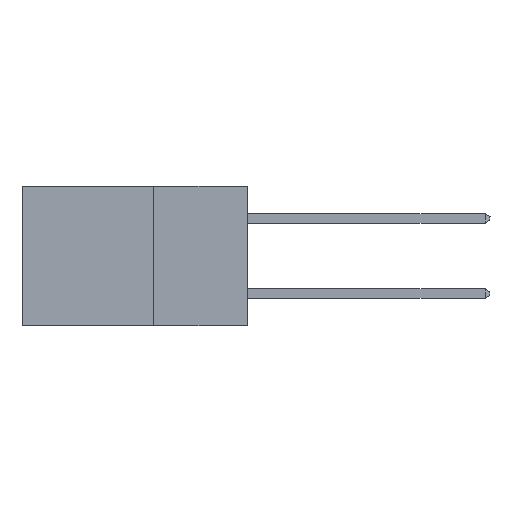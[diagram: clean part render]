
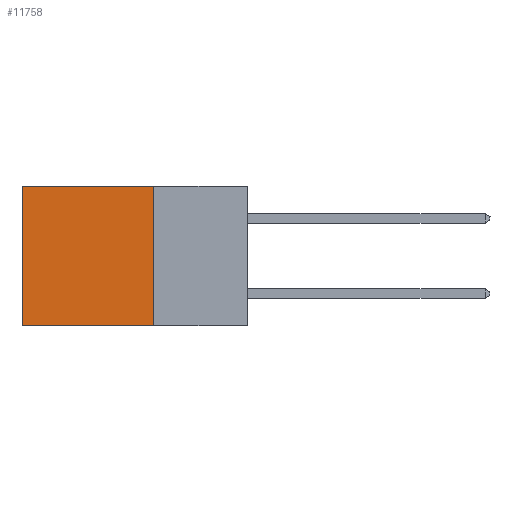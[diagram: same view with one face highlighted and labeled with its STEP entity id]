
A CAD part, left-side view. The second image highlights one B-rep face of the part: STEP entity #11758.
In plain terms, the highlighted planar face has unit normal (-1, 0, 0).
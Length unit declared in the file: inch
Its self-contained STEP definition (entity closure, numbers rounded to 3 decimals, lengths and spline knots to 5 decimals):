
#972 = DIRECTION ( 'NONE',  ( 0., 0., -1. ) ) ;
#1285 = EDGE_CURVE ( 'NONE', #8118, #17731, #5381, .T. ) ;
#1429 = LINE ( 'NONE', #10529, #5574 ) ;
#1528 = CARTESIAN_POINT ( 'NONE',  ( 0.2615, 0.25, 0. ) ) ;
#1572 = DIRECTION ( 'NONE',  ( 0., 0., -1. ) ) ;
#1685 = ORIENTED_EDGE ( 'NONE', *, *, #16047, .F. ) ;
#2729 = DIRECTION ( 'NONE',  ( 0., 1., 0. ) ) ;
#2750 = VECTOR ( 'NONE', #16886, 39.37008 ) ;
#2958 = PLANE ( 'NONE',  #10646 ) ;
#3011 = DIRECTION ( 'NONE',  ( 0., 1., 0. ) ) ;
#3368 = VERTEX_POINT ( 'NONE', #1528 ) ;
#3438 = EDGE_CURVE ( 'NONE', #3368, #5567, #10914, .T. ) ;
#4516 = CARTESIAN_POINT ( 'NONE',  ( 0.2615, 0.25, -0.37 ) ) ;
#5381 = LINE ( 'NONE', #16934, #14533 ) ;
#5567 = VERTEX_POINT ( 'NONE', #5978 ) ;
#5574 = VECTOR ( 'NONE', #3011, 39.37008 ) ;
#5978 = CARTESIAN_POINT ( 'NONE',  ( 0.2615, 0.25, -0.37 ) ) ;
#7473 = CARTESIAN_POINT ( 'NONE',  ( 0.2615, 0.6, -0.37 ) ) ;
#8118 = VERTEX_POINT ( 'NONE', #16156 ) ;
#8455 = ORIENTED_EDGE ( 'NONE', *, *, #3438, .F. ) ;
#8831 = FACE_OUTER_BOUND ( 'NONE', #18727, .T. ) ;
#10159 = CARTESIAN_POINT ( 'NONE',  ( 0.2615, 0.25, 0. ) ) ;
#10181 = DIRECTION ( 'NONE',  ( 1., 0., 0. ) ) ;
#10529 = CARTESIAN_POINT ( 'NONE',  ( 0.2615, 0.25, -0.37 ) ) ;
#10646 = AXIS2_PLACEMENT_3D ( 'NONE', #4516, #10181, #1572 ) ;
#10914 = LINE ( 'NONE', #18470, #2750 ) ;
#11339 = LINE ( 'NONE', #10159, #18526 ) ;
#11758 = ADVANCED_FACE ( 'NONE', ( #8831 ), #2958, .F. ) ;
#13925 = EDGE_CURVE ( 'NONE', #3368, #8118, #11339, .T. ) ;
#14533 = VECTOR ( 'NONE', #972, 39.37008 ) ;
#16047 = EDGE_CURVE ( 'NONE', #5567, #17731, #1429, .T. ) ;
#16156 = CARTESIAN_POINT ( 'NONE',  ( 0.2615, 0.6, 0. ) ) ;
#16886 = DIRECTION ( 'NONE',  ( 0., 0., -1. ) ) ;
#16934 = CARTESIAN_POINT ( 'NONE',  ( 0.2615, 0.6, -0.37 ) ) ;
#16984 = ORIENTED_EDGE ( 'NONE', *, *, #1285, .T. ) ;
#17731 = VERTEX_POINT ( 'NONE', #7473 ) ;
#17805 = ORIENTED_EDGE ( 'NONE', *, *, #13925, .T. ) ;
#18470 = CARTESIAN_POINT ( 'NONE',  ( 0.2615, 0.25, -0.37 ) ) ;
#18526 = VECTOR ( 'NONE', #2729, 39.37008 ) ;
#18727 = EDGE_LOOP ( 'NONE', ( #16984, #1685, #8455, #17805 ) ) ;
